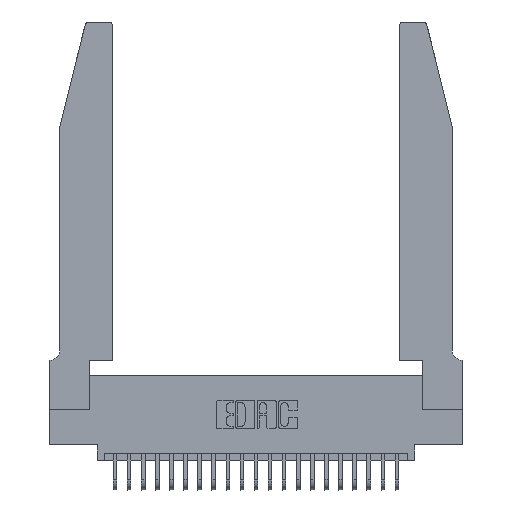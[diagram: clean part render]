
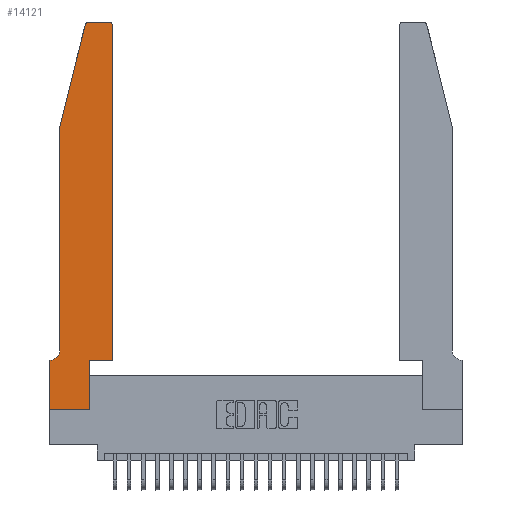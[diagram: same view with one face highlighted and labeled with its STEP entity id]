
A CAD part, top view. The second image highlights one B-rep face of the part: STEP entity #14121.
In plain terms, the highlighted planar face has unit normal (0, 0, 1).
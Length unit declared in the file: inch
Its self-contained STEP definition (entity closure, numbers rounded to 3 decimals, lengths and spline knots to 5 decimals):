
#531 = EDGE_CURVE ( 'NONE', #14023, #8211, #23468, .T. ) ;
#557 = EDGE_CURVE ( 'NONE', #20128, #9096, #12514, .T. ) ;
#670 = DIRECTION ( 'NONE',  ( 1., 0., 0. ) ) ;
#1213 = LINE ( 'NONE', #5184, #16853 ) ;
#1384 = DIRECTION ( 'NONE',  ( 1., 0., 0. ) ) ;
#1615 = CARTESIAN_POINT ( 'NONE',  ( 0.2865, 0.35, 0.37 ) ) ;
#2150 = EDGE_CURVE ( 'NONE', #8211, #2640, #16507, .T. ) ;
#2463 = LINE ( 'NONE', #14641, #7315 ) ;
#2640 = VERTEX_POINT ( 'NONE', #15871 ) ;
#2803 = CIRCLE ( 'NONE', #15928, 0.03 ) ;
#2846 = VECTOR ( 'NONE', #10942, 39.37008 ) ;
#3045 = VECTOR ( 'NONE', #15929, 39.37008 ) ;
#4174 = DIRECTION ( 'NONE',  ( 0., -1., 0. ) ) ;
#5157 = DIRECTION ( 'NONE',  ( -1., 0., 0. ) ) ;
#5184 = CARTESIAN_POINT ( 'NONE',  ( 0.4505, 0.35, 0.37 ) ) ;
#5251 = ORIENTED_EDGE ( 'NONE', *, *, #12129, .T. ) ;
#5707 = ORIENTED_EDGE ( 'NONE', *, *, #11990, .T. ) ;
#5753 = CARTESIAN_POINT ( 'NONE',  ( 0.4505, 2.72, 0.37 ) ) ;
#6154 = ORIENTED_EDGE ( 'NONE', *, *, #17761, .T. ) ;
#6464 = ORIENTED_EDGE ( 'NONE', *, *, #25169, .T. ) ;
#6487 = CARTESIAN_POINT ( 'NONE',  ( 0., 0.35, 0.37 ) ) ;
#6782 = CIRCLE ( 'NONE', #25303, 0.07 ) ;
#7036 = VERTEX_POINT ( 'NONE', #25859 ) ;
#7056 = VECTOR ( 'NONE', #1384, 39.37008 ) ;
#7315 = VECTOR ( 'NONE', #14730, 39.37008 ) ;
#7817 = DIRECTION ( 'NONE',  ( 0., -1., 0. ) ) ;
#8004 = CARTESIAN_POINT ( 'NONE',  ( 0., 0., 0.37 ) ) ;
#8211 = VERTEX_POINT ( 'NONE', #5753 ) ;
#8347 = DIRECTION ( 'NONE',  ( 0., 0., -1. ) ) ;
#8600 = ORIENTED_EDGE ( 'NONE', *, *, #17994, .T. ) ;
#9096 = VERTEX_POINT ( 'NONE', #10318 ) ;
#9447 = LINE ( 'NONE', #18347, #23277 ) ;
#9780 = ORIENTED_EDGE ( 'NONE', *, *, #13953, .T. ) ;
#9873 = DIRECTION ( 'NONE',  ( 0., 0., 1. ) ) ;
#9907 = VERTEX_POINT ( 'NONE', #10459 ) ;
#10016 = ORIENTED_EDGE ( 'NONE', *, *, #557, .T. ) ;
#10221 = DIRECTION ( 'NONE',  ( 0., 0., 1. ) ) ;
#10256 = CARTESIAN_POINT ( 'NONE',  ( 0.4505, 0.35, 0.37 ) ) ;
#10260 = ORIENTED_EDGE ( 'NONE', *, *, #2150, .T. ) ;
#10318 = CARTESIAN_POINT ( 'NONE',  ( 0.2865, 0., 0.37 ) ) ;
#10459 = CARTESIAN_POINT ( 'NONE',  ( 0.0055, 0.35, 0.37 ) ) ;
#10942 = DIRECTION ( 'NONE',  ( 0., 1., 0. ) ) ;
#11694 = VERTEX_POINT ( 'NONE', #6487 ) ;
#11990 = EDGE_CURVE ( 'NONE', #11694, #20128, #19956, .T. ) ;
#12129 = EDGE_CURVE ( 'NONE', #25223, #9907, #6782, .T. ) ;
#12475 = VECTOR ( 'NONE', #5157, 39.37008 ) ;
#12514 = LINE ( 'NONE', #8004, #7056 ) ;
#12941 = CARTESIAN_POINT ( 'NONE',  ( 0.25487, 2.72718, 0.37 ) ) ;
#12989 = DIRECTION ( 'NONE',  ( 0., 0., 1. ) ) ;
#13948 = LINE ( 'NONE', #1615, #3045 ) ;
#13953 = EDGE_CURVE ( 'NONE', #7036, #25223, #9447, .T. ) ;
#14023 = VERTEX_POINT ( 'NONE', #24190 ) ;
#14121 = ADVANCED_FACE ( 'NONE', ( #25116 ), #24619, .T. ) ;
#14641 = CARTESIAN_POINT ( 'NONE',  ( 0.0755, 0.35, 0.37 ) ) ;
#14730 = DIRECTION ( 'NONE',  ( -1., 0., 0. ) ) ;
#14760 = LINE ( 'NONE', #15579, #18722 ) ;
#14883 = CARTESIAN_POINT ( 'NONE',  ( 0.2865, 0.35, 0.37 ) ) ;
#15361 = CARTESIAN_POINT ( 'NONE',  ( 0.2605, 2.75, 0.37 ) ) ;
#15579 = CARTESIAN_POINT ( 'NONE',  ( 0.0755, 2., 0.37 ) ) ;
#15695 = AXIS2_PLACEMENT_3D ( 'NONE', #22008, #10221, #23916 ) ;
#15871 = CARTESIAN_POINT ( 'NONE',  ( 0.4205, 2.75, 0.37 ) ) ;
#15928 = AXIS2_PLACEMENT_3D ( 'NONE', #21692, #9873, #23605 ) ;
#15929 = DIRECTION ( 'NONE',  ( 0., 1., 0. ) ) ;
#16507 = CIRCLE ( 'NONE', #15695, 0.03 ) ;
#16853 = VECTOR ( 'NONE', #21207, 39.37008 ) ;
#16913 = CARTESIAN_POINT ( 'NONE',  ( 0., 0.35, 0.37 ) ) ;
#17585 = EDGE_CURVE ( 'NONE', #20814, #14023, #1213, .T. ) ;
#17753 = LINE ( 'NONE', #15361, #12475 ) ;
#17761 = EDGE_CURVE ( 'NONE', #18072, #19032, #2803, .T. ) ;
#17994 = EDGE_CURVE ( 'NONE', #9907, #11694, #2463, .T. ) ;
#18072 = VERTEX_POINT ( 'NONE', #24850 ) ;
#18347 = CARTESIAN_POINT ( 'NONE',  ( 0.0755, 2., 0.37 ) ) ;
#18604 = AXIS2_PLACEMENT_3D ( 'NONE', #16913, #12989, #670 ) ;
#18722 = VECTOR ( 'NONE', #21391, 39.37008 ) ;
#18956 = ORIENTED_EDGE ( 'NONE', *, *, #531, .T. ) ;
#19032 = VERTEX_POINT ( 'NONE', #12941 ) ;
#19363 = ORIENTED_EDGE ( 'NONE', *, *, #19386, .T. ) ;
#19386 = EDGE_CURVE ( 'NONE', #9096, #20814, #13948, .T. ) ;
#19956 = LINE ( 'NONE', #21718, #21153 ) ;
#20128 = VERTEX_POINT ( 'NONE', #22353 ) ;
#20286 = CARTESIAN_POINT ( 'NONE',  ( 0.0055, 0.42, 0.37 ) ) ;
#20592 = ORIENTED_EDGE ( 'NONE', *, *, #17585, .T. ) ;
#20814 = VERTEX_POINT ( 'NONE', #14883 ) ;
#21153 = VECTOR ( 'NONE', #7817, 39.37008 ) ;
#21207 = DIRECTION ( 'NONE',  ( 1., 0., 0. ) ) ;
#21391 = DIRECTION ( 'NONE',  ( -0.239, -0.971, 0. ) ) ;
#21692 = CARTESIAN_POINT ( 'NONE',  ( 0.284, 2.72, 0.37 ) ) ;
#21718 = CARTESIAN_POINT ( 'NONE',  ( 0., 0., 0.37 ) ) ;
#22008 = CARTESIAN_POINT ( 'NONE',  ( 0.4205, 2.72, 0.37 ) ) ;
#22202 = DIRECTION ( 'NONE',  ( -1., 0., 0. ) ) ;
#22353 = CARTESIAN_POINT ( 'NONE',  ( 0., 0., 0.37 ) ) ;
#23168 = CARTESIAN_POINT ( 'NONE',  ( 0.0755, 0.42, 0.37 ) ) ;
#23277 = VECTOR ( 'NONE', #4174, 39.37008 ) ;
#23468 = LINE ( 'NONE', #10256, #2846 ) ;
#23540 = EDGE_CURVE ( 'NONE', #19032, #7036, #14760, .T. ) ;
#23605 = DIRECTION ( 'NONE',  ( 1., 0., 0. ) ) ;
#23916 = DIRECTION ( 'NONE',  ( 1., 0., 0. ) ) ;
#24190 = CARTESIAN_POINT ( 'NONE',  ( 0.4505, 0.35, 0.37 ) ) ;
#24544 = ORIENTED_EDGE ( 'NONE', *, *, #23540, .T. ) ;
#24590 = EDGE_LOOP ( 'NONE', ( #6464, #6154, #24544, #9780, #5251, #8600, #5707, #10016, #19363, #20592, #18956, #10260 ) ) ;
#24619 = PLANE ( 'NONE',  #18604 ) ;
#24850 = CARTESIAN_POINT ( 'NONE',  ( 0.284, 2.75, 0.37 ) ) ;
#25116 = FACE_OUTER_BOUND ( 'NONE', #24590, .T. ) ;
#25169 = EDGE_CURVE ( 'NONE', #2640, #18072, #17753, .T. ) ;
#25223 = VERTEX_POINT ( 'NONE', #23168 ) ;
#25303 = AXIS2_PLACEMENT_3D ( 'NONE', #20286, #8347, #22202 ) ;
#25859 = CARTESIAN_POINT ( 'NONE',  ( 0.0755, 2., 0.37 ) ) ;
